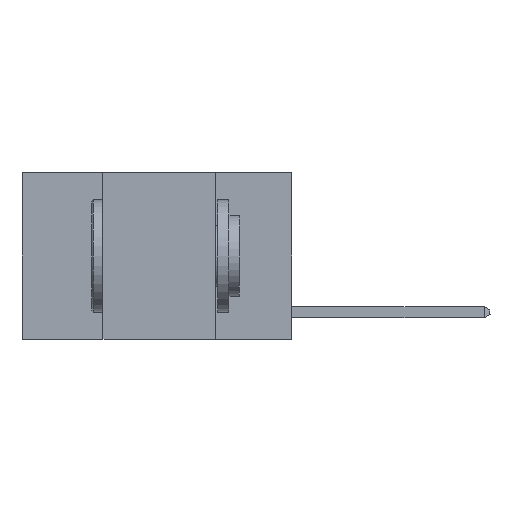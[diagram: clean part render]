
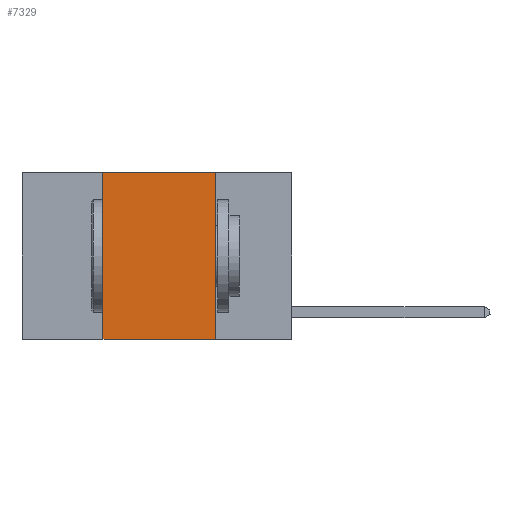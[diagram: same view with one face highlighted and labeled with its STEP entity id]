
A CAD part, left-side view. The second image highlights one B-rep face of the part: STEP entity #7329.
In plain terms, the highlighted planar face has unit normal (-1, 0, 0).
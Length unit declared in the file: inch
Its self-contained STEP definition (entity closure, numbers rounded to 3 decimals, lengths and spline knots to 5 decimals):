
#13 = CARTESIAN_POINT ( 'NONE',  ( 0., 0.17, -0.37 ) ) ;
#1367 = EDGE_CURVE ( 'NONE', #4899, #17161, #15512, .T. ) ;
#1481 = CARTESIAN_POINT ( 'NONE',  ( 0., 0.17, 0. ) ) ;
#2314 = EDGE_CURVE ( 'NONE', #4899, #17595, #13675, .T. ) ;
#2589 = AXIS2_PLACEMENT_3D ( 'NONE', #3886, #16868, #8199 ) ;
#2693 = FACE_OUTER_BOUND ( 'NONE', #8401, .T. ) ;
#3284 = EDGE_CURVE ( 'NONE', #17595, #8743, #15016, .T. ) ;
#3886 = CARTESIAN_POINT ( 'NONE',  ( 0., 0.6, 0. ) ) ;
#4062 = CARTESIAN_POINT ( 'NONE',  ( 0., 0.17, 0. ) ) ;
#4272 = CARTESIAN_POINT ( 'NONE',  ( 0., 0.6, -0.37 ) ) ;
#4406 = DIRECTION ( 'NONE',  ( 0., -1., 0. ) ) ;
#4885 = ORIENTED_EDGE ( 'NONE', *, *, #2314, .F. ) ;
#4899 = VERTEX_POINT ( 'NONE', #13560 ) ;
#5190 = CARTESIAN_POINT ( 'NONE',  ( 0., 0.42, 0. ) ) ;
#5328 = ORIENTED_EDGE ( 'NONE', *, *, #1367, .T. ) ;
#6744 = PLANE ( 'NONE',  #2589 ) ;
#7205 = DIRECTION ( 'NONE',  ( 0., 0., -1. ) ) ;
#7329 = ADVANCED_FACE ( 'NONE', ( #2693 ), #6744, .F. ) ;
#8165 = VECTOR ( 'NONE', #7205, 39.37008 ) ;
#8199 = DIRECTION ( 'NONE',  ( 0., 0., -1. ) ) ;
#8220 = ORIENTED_EDGE ( 'NONE', *, *, #16787, .F. ) ;
#8401 = EDGE_LOOP ( 'NONE', ( #8220, #12102, #4885, #5328 ) ) ;
#8743 = VERTEX_POINT ( 'NONE', #4062 ) ;
#9145 = CARTESIAN_POINT ( 'NONE',  ( 0., 0.42, 0. ) ) ;
#11167 = VECTOR ( 'NONE', #15875, 39.37008 ) ;
#12102 = ORIENTED_EDGE ( 'NONE', *, *, #3284, .F. ) ;
#13560 = CARTESIAN_POINT ( 'NONE',  ( 0., 0.42, -0.37 ) ) ;
#13675 = LINE ( 'NONE', #9145, #17950 ) ;
#14443 = CARTESIAN_POINT ( 'NONE',  ( 0., 0.6, 0. ) ) ;
#15016 = LINE ( 'NONE', #14443, #11167 ) ;
#15512 = LINE ( 'NONE', #4272, #15952 ) ;
#15875 = DIRECTION ( 'NONE',  ( 0., -1., 0. ) ) ;
#15876 = LINE ( 'NONE', #1481, #8165 ) ;
#15952 = VECTOR ( 'NONE', #4406, 39.37008 ) ;
#16787 = EDGE_CURVE ( 'NONE', #8743, #17161, #15876, .T. ) ;
#16868 = DIRECTION ( 'NONE',  ( 1., 0., 0. ) ) ;
#17161 = VERTEX_POINT ( 'NONE', #13 ) ;
#17595 = VERTEX_POINT ( 'NONE', #5190 ) ;
#17806 = DIRECTION ( 'NONE',  ( 0., 0., 1. ) ) ;
#17950 = VECTOR ( 'NONE', #17806, 39.37008 ) ;
